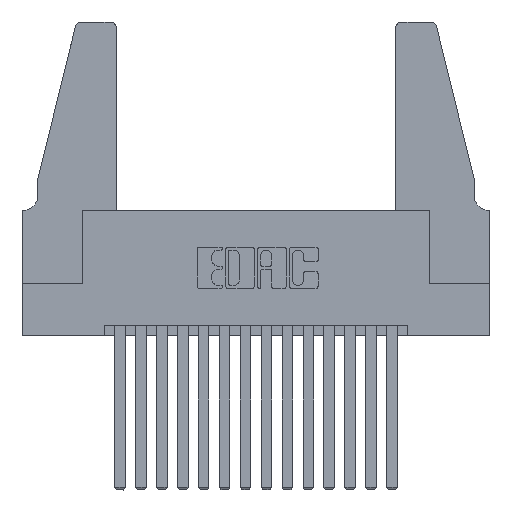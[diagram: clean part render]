
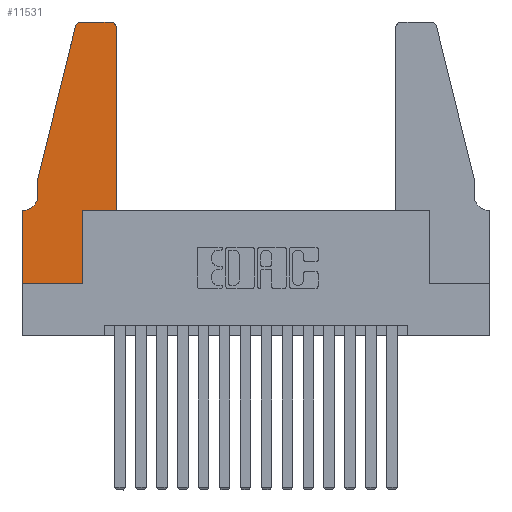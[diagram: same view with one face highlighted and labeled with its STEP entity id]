
A CAD part, top view. The second image highlights one B-rep face of the part: STEP entity #11531.
In plain terms, the highlighted planar face has unit normal (0, 0, 1).
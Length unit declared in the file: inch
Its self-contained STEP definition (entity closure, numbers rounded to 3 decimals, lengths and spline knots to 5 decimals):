
#199 = DIRECTION ( 'NONE',  ( -1., 0., 0. ) ) ;
#383 = ORIENTED_EDGE ( 'NONE', *, *, #3128, .T. ) ;
#394 = EDGE_CURVE ( 'NONE', #7113, #8927, #5869, .T. ) ;
#405 = ORIENTED_EDGE ( 'NONE', *, *, #394, .T. ) ;
#664 = ORIENTED_EDGE ( 'NONE', *, *, #5619, .T. ) ;
#907 = CARTESIAN_POINT ( 'NONE',  ( 0., 0., 0.37 ) ) ;
#928 = LINE ( 'NONE', #14309, #13450 ) ;
#953 = VECTOR ( 'NONE', #14821, 39.37008 ) ;
#1121 = VECTOR ( 'NONE', #1833, 39.37008 ) ;
#1388 = VERTEX_POINT ( 'NONE', #15072 ) ;
#1461 = VERTEX_POINT ( 'NONE', #907 ) ;
#1742 = VECTOR ( 'NONE', #16551, 39.37008 ) ;
#1791 = LINE ( 'NONE', #6989, #13697 ) ;
#1801 = VERTEX_POINT ( 'NONE', #3147 ) ;
#1833 = DIRECTION ( 'NONE',  ( -0.239, -0.971, 0. ) ) ;
#1836 = VERTEX_POINT ( 'NONE', #5786 ) ;
#1838 = CARTESIAN_POINT ( 'NONE',  ( 0.2865, 0.35, 0.37 ) ) ;
#1842 = DIRECTION ( 'NONE',  ( 0., 1., 0. ) ) ;
#1925 = DIRECTION ( 'NONE',  ( 1., 0., 0. ) ) ;
#1943 = ORIENTED_EDGE ( 'NONE', *, *, #8487, .T. ) ;
#2090 = VECTOR ( 'NONE', #10401, 39.37008 ) ;
#2143 = LINE ( 'NONE', #13688, #1121 ) ;
#2499 = CARTESIAN_POINT ( 'NONE',  ( 0.4205, 1.25, 0.37 ) ) ;
#2588 = CARTESIAN_POINT ( 'NONE',  ( 0.0755, 0.35, 0.37 ) ) ;
#2695 = DIRECTION ( 'NONE',  ( 0., -1., 0. ) ) ;
#2704 = EDGE_CURVE ( 'NONE', #1801, #1836, #1791, .T. ) ;
#2764 = DIRECTION ( 'NONE',  ( 1., 0., 0. ) ) ;
#2968 = CARTESIAN_POINT ( 'NONE',  ( 0.4505, 0.35, 0.37 ) ) ;
#3128 = EDGE_CURVE ( 'NONE', #7389, #6471, #3397, .T. ) ;
#3147 = CARTESIAN_POINT ( 'NONE',  ( 0.0755, 0.5, 0.37 ) ) ;
#3397 = LINE ( 'NONE', #1838, #953 ) ;
#3571 = AXIS2_PLACEMENT_3D ( 'NONE', #5072, #6367, #8931 ) ;
#3960 = CARTESIAN_POINT ( 'NONE',  ( 0.2865, 0., 0.37 ) ) ;
#4089 = CARTESIAN_POINT ( 'NONE',  ( 0.284, 1.25, 0.37 ) ) ;
#4425 = VECTOR ( 'NONE', #1842, 39.37008 ) ;
#4696 = LINE ( 'NONE', #2588, #2090 ) ;
#5072 = CARTESIAN_POINT ( 'NONE',  ( 0.284, 1.22, 0.37 ) ) ;
#5470 = EDGE_LOOP ( 'NONE', ( #405, #12126, #11149, #14401, #16124, #1943, #664, #8519, #383, #9807, #16071, #13931 ) ) ;
#5619 = EDGE_CURVE ( 'NONE', #7606, #1461, #928, .T. ) ;
#5761 = EDGE_CURVE ( 'NONE', #1461, #7389, #9574, .T. ) ;
#5786 = CARTESIAN_POINT ( 'NONE',  ( 0.0755, 0.42, 0.37 ) ) ;
#5869 = LINE ( 'NONE', #15630, #14960 ) ;
#5989 = FACE_OUTER_BOUND ( 'NONE', #5470, .T. ) ;
#6352 = CARTESIAN_POINT ( 'NONE',  ( 0.2865, 0.35, 0.37 ) ) ;
#6367 = DIRECTION ( 'NONE',  ( 0., 0., 1. ) ) ;
#6421 = CIRCLE ( 'NONE', #9386, 0.03 ) ;
#6455 = DIRECTION ( 'NONE',  ( 0., 0., 1. ) ) ;
#6471 = VERTEX_POINT ( 'NONE', #6352 ) ;
#6989 = CARTESIAN_POINT ( 'NONE',  ( 0.0755, 0.5, 0.37 ) ) ;
#7113 = VERTEX_POINT ( 'NONE', #2499 ) ;
#7141 = CARTESIAN_POINT ( 'NONE',  ( 0.0055, 0.42, 0.37 ) ) ;
#7292 = VERTEX_POINT ( 'NONE', #13102 ) ;
#7306 = DIRECTION ( 'NONE',  ( -1., 0., 0. ) ) ;
#7330 = VECTOR ( 'NONE', #1925, 39.37008 ) ;
#7389 = VERTEX_POINT ( 'NONE', #3960 ) ;
#7606 = VERTEX_POINT ( 'NONE', #14949 ) ;
#7915 = CARTESIAN_POINT ( 'NONE',  ( 0.0055, 0.35, 0.37 ) ) ;
#7927 = DIRECTION ( 'NONE',  ( 0., 0., 1. ) ) ;
#8105 = EDGE_CURVE ( 'NONE', #1836, #8583, #10346, .T. ) ;
#8487 = EDGE_CURVE ( 'NONE', #8583, #7606, #4696, .T. ) ;
#8519 = ORIENTED_EDGE ( 'NONE', *, *, #5761, .T. ) ;
#8536 = LINE ( 'NONE', #12983, #7330 ) ;
#8583 = VERTEX_POINT ( 'NONE', #7915 ) ;
#8927 = VERTEX_POINT ( 'NONE', #4089 ) ;
#8931 = DIRECTION ( 'NONE',  ( 1., 0., 0. ) ) ;
#9386 = AXIS2_PLACEMENT_3D ( 'NONE', #10512, #6455, #14200 ) ;
#9574 = LINE ( 'NONE', #16497, #1742 ) ;
#9807 = ORIENTED_EDGE ( 'NONE', *, *, #13267, .T. ) ;
#10346 = CIRCLE ( 'NONE', #13927, 0.07 ) ;
#10350 = CARTESIAN_POINT ( 'NONE',  ( 0., 0.35, 0.37 ) ) ;
#10401 = DIRECTION ( 'NONE',  ( -1., 0., 0. ) ) ;
#10512 = CARTESIAN_POINT ( 'NONE',  ( 0.4205, 1.22, 0.37 ) ) ;
#10571 = EDGE_CURVE ( 'NONE', #14178, #1388, #12290, .T. ) ;
#10792 = CARTESIAN_POINT ( 'NONE',  ( 0.4505, 0.35, 0.37 ) ) ;
#11149 = ORIENTED_EDGE ( 'NONE', *, *, #12402, .T. ) ;
#11267 = AXIS2_PLACEMENT_3D ( 'NONE', #10350, #7927, #2764 ) ;
#11531 = ADVANCED_FACE ( 'NONE', ( #5989 ), #15637, .T. ) ;
#11775 = CIRCLE ( 'NONE', #3571, 0.03 ) ;
#12081 = DIRECTION ( 'NONE',  ( 0., -1., 0. ) ) ;
#12126 = ORIENTED_EDGE ( 'NONE', *, *, #13360, .T. ) ;
#12290 = LINE ( 'NONE', #10792, #4425 ) ;
#12402 = EDGE_CURVE ( 'NONE', #7292, #1801, #2143, .T. ) ;
#12983 = CARTESIAN_POINT ( 'NONE',  ( 0.4505, 0.35, 0.37 ) ) ;
#13102 = CARTESIAN_POINT ( 'NONE',  ( 0.25487, 1.22718, 0.37 ) ) ;
#13267 = EDGE_CURVE ( 'NONE', #6471, #14178, #8536, .T. ) ;
#13360 = EDGE_CURVE ( 'NONE', #8927, #7292, #11775, .T. ) ;
#13450 = VECTOR ( 'NONE', #2695, 39.37008 ) ;
#13688 = CARTESIAN_POINT ( 'NONE',  ( 0.0755, 0.5, 0.37 ) ) ;
#13697 = VECTOR ( 'NONE', #12081, 39.37008 ) ;
#13927 = AXIS2_PLACEMENT_3D ( 'NONE', #7141, #14940, #7306 ) ;
#13931 = ORIENTED_EDGE ( 'NONE', *, *, #16471, .T. ) ;
#14178 = VERTEX_POINT ( 'NONE', #2968 ) ;
#14200 = DIRECTION ( 'NONE',  ( 1., 0., 0. ) ) ;
#14309 = CARTESIAN_POINT ( 'NONE',  ( 0., 0., 0.37 ) ) ;
#14401 = ORIENTED_EDGE ( 'NONE', *, *, #2704, .T. ) ;
#14821 = DIRECTION ( 'NONE',  ( 0., 1., 0. ) ) ;
#14940 = DIRECTION ( 'NONE',  ( 0., 0., -1. ) ) ;
#14949 = CARTESIAN_POINT ( 'NONE',  ( 0., 0.35, 0.37 ) ) ;
#14960 = VECTOR ( 'NONE', #199, 39.37008 ) ;
#15072 = CARTESIAN_POINT ( 'NONE',  ( 0.4505, 1.22, 0.37 ) ) ;
#15630 = CARTESIAN_POINT ( 'NONE',  ( 0.2605, 1.25, 0.37 ) ) ;
#15637 = PLANE ( 'NONE',  #11267 ) ;
#16071 = ORIENTED_EDGE ( 'NONE', *, *, #10571, .T. ) ;
#16124 = ORIENTED_EDGE ( 'NONE', *, *, #8105, .T. ) ;
#16471 = EDGE_CURVE ( 'NONE', #1388, #7113, #6421, .T. ) ;
#16497 = CARTESIAN_POINT ( 'NONE',  ( 0., 0., 0.37 ) ) ;
#16551 = DIRECTION ( 'NONE',  ( 1., 0., 0. ) ) ;
